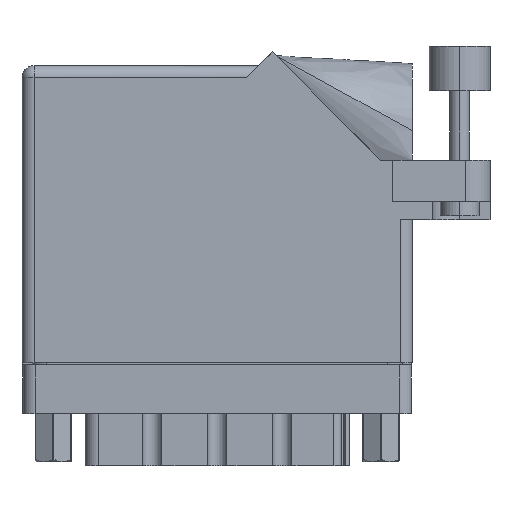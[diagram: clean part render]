
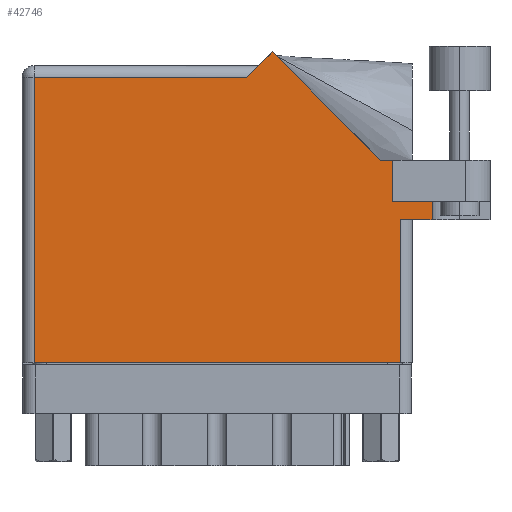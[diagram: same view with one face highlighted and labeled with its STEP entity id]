
A CAD part, front view. The second image highlights one B-rep face of the part: STEP entity #42746.
In plain terms, the highlighted face is planar.
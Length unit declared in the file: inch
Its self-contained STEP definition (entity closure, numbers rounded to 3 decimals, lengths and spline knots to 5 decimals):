
#1535 = CARTESIAN_POINT ( 'NONE',  ( 1.155, 1.468, 0. ) ) ;
#1618 = VECTOR ( 'NONE', #23216, 39.37008 ) ;
#1733 = PLANE ( 'NONE',  #25027 ) ;
#2465 = CARTESIAN_POINT ( 'NONE',  ( 1.217, 1.53, 0. ) ) ;
#3577 = VECTOR ( 'NONE', #14190, 39.37008 ) ;
#3691 = CARTESIAN_POINT ( 'NONE',  ( 1.84442, 1.044, 0. ) ) ;
#4006 = LINE ( 'NONE', #43678, #33752 ) ;
#4543 = VERTEX_POINT ( 'NONE', #36850 ) ;
#5243 = DIRECTION ( 'NONE',  ( -1., 0., 0. ) ) ;
#6204 = EDGE_CURVE ( 'NONE', #18071, #45854, #47728, .T. ) ;
#6948 = EDGE_CURVE ( 'NONE', #42936, #18071, #4006, .T. ) ;
#7545 = ORIENTED_EDGE ( 'NONE', *, *, #11452, .T. ) ;
#8191 = ORIENTED_EDGE ( 'NONE', *, *, #13982, .T. ) ;
#8495 = VECTOR ( 'NONE', #10688, 39.37008 ) ;
#9324 = ORIENTED_EDGE ( 'NONE', *, *, #23340, .F. ) ;
#9663 = LINE ( 'NONE', #29232, #18688 ) ;
#10382 = CARTESIAN_POINT ( 'NONE',  ( 2.1115, 1.16177, 0. ) ) ;
#10423 = VECTOR ( 'NONE', #29510, 39.37008 ) ;
#10688 = DIRECTION ( 'NONE',  ( 0., -1., 0. ) ) ;
#10839 = CARTESIAN_POINT ( 'NONE',  ( 0., 0., 0. ) ) ;
#11452 = EDGE_CURVE ( 'NONE', #45854, #25135, #19325, .T. ) ;
#12275 = EDGE_CURVE ( 'NONE', #35426, #27880, #9663, .T. ) ;
#13713 = DIRECTION ( 'NONE',  ( -1., 0., 0. ) ) ;
#13982 = EDGE_CURVE ( 'NONE', #35426, #42936, #41427, .T. ) ;
#14123 = DIRECTION ( 'NONE',  ( 0., 0., -1. ) ) ;
#14190 = DIRECTION ( 'NONE',  ( -0.707, -0.707, 0. ) ) ;
#15626 = CARTESIAN_POINT ( 'NONE',  ( 2.1115, 0.737, 0. ) ) ;
#17473 = VECTOR ( 'NONE', #19824, 39.37008 ) ;
#17929 = VECTOR ( 'NONE', #42366, 39.37008 ) ;
#17987 = DIRECTION ( 'NONE',  ( -1., 0., 0. ) ) ;
#18071 = VERTEX_POINT ( 'NONE', #38357 ) ;
#18688 = VECTOR ( 'NONE', #44945, 39.37008 ) ;
#19325 = LINE ( 'NONE', #2465, #3577 ) ;
#19680 = ORIENTED_EDGE ( 'NONE', *, *, #31225, .T. ) ;
#19824 = DIRECTION ( 'NONE',  ( 0., 1., 0. ) ) ;
#19980 = CARTESIAN_POINT ( 'NONE',  ( 1.91, 0.831, 0. ) ) ;
#21024 = EDGE_CURVE ( 'NONE', #4543, #29159, #24658, .T. ) ;
#22204 = ORIENTED_EDGE ( 'NONE', *, *, #6204, .T. ) ;
#23216 = DIRECTION ( 'NONE',  ( -0.707, 0.707, 0. ) ) ;
#23340 = EDGE_CURVE ( 'NONE', #27880, #29159, #29975, .T. ) ;
#24658 = LINE ( 'NONE', #46274, #17929 ) ;
#24709 = FACE_OUTER_BOUND ( 'NONE', #35248, .T. ) ;
#25027 = AXIS2_PLACEMENT_3D ( 'NONE', #32777, #14123, #17987 ) ;
#25135 = VERTEX_POINT ( 'NONE', #1535 ) ;
#25225 = EDGE_CURVE ( 'NONE', #42464, #33213, #40710, .T. ) ;
#26280 = CARTESIAN_POINT ( 'NONE',  ( 0., 1.468, 0. ) ) ;
#27232 = LINE ( 'NONE', #26280, #27827 ) ;
#27825 = CARTESIAN_POINT ( 'NONE',  ( 0.062, 0., 0. ) ) ;
#27827 = VECTOR ( 'NONE', #13713, 39.37008 ) ;
#27880 = VERTEX_POINT ( 'NONE', #39480 ) ;
#27953 = CARTESIAN_POINT ( 'NONE',  ( 0.062, 0., 0. ) ) ;
#28013 = CARTESIAN_POINT ( 'NONE',  ( 1.91, 0.831, 0. ) ) ;
#29159 = VERTEX_POINT ( 'NONE', #15626 ) ;
#29232 = CARTESIAN_POINT ( 'NONE',  ( 1.91, 0.831, 0. ) ) ;
#29402 = ORIENTED_EDGE ( 'NONE', *, *, #41650, .T. ) ;
#29510 = DIRECTION ( 'NONE',  ( 1., 0., 0. ) ) ;
#29975 = LINE ( 'NONE', #10382, #40800 ) ;
#30080 = CARTESIAN_POINT ( 'NONE',  ( 1.91, 1.044, 0. ) ) ;
#30337 = ORIENTED_EDGE ( 'NONE', *, *, #21024, .T. ) ;
#30879 = CARTESIAN_POINT ( 'NONE',  ( 1.28771, 1.60071, 0. ) ) ;
#31225 = EDGE_CURVE ( 'NONE', #38385, #42464, #44227, .T. ) ;
#31890 = ORIENTED_EDGE ( 'NONE', *, *, #25225, .T. ) ;
#32777 = CARTESIAN_POINT ( 'NONE',  ( 0., 1.53, 0. ) ) ;
#33213 = VERTEX_POINT ( 'NONE', #44200 ) ;
#33576 = DIRECTION ( 'NONE',  ( 0., -1., 0. ) ) ;
#33752 = VECTOR ( 'NONE', #5243, 39.37008 ) ;
#34679 = CARTESIAN_POINT ( 'NONE',  ( 0.062, 1.468, 0. ) ) ;
#35248 = EDGE_LOOP ( 'NONE', ( #31890, #38006, #30337, #9324, #44285, #8191, #39611, #22204, #7545, #29402, #19680 ) ) ;
#35426 = VERTEX_POINT ( 'NONE', #19980 ) ;
#35747 = CARTESIAN_POINT ( 'NONE',  ( 1.948, 0.737, 0. ) ) ;
#36850 = CARTESIAN_POINT ( 'NONE',  ( 1.948, 0.737, 0. ) ) ;
#37785 = VECTOR ( 'NONE', #47267, 39.37008 ) ;
#38006 = ORIENTED_EDGE ( 'NONE', *, *, #41460, .T. ) ;
#38357 = CARTESIAN_POINT ( 'NONE',  ( 1.84442, 1.044, 0. ) ) ;
#38385 = VERTEX_POINT ( 'NONE', #34679 ) ;
#39480 = CARTESIAN_POINT ( 'NONE',  ( 2.1115, 0.831, 0. ) ) ;
#39611 = ORIENTED_EDGE ( 'NONE', *, *, #6948, .T. ) ;
#40710 = LINE ( 'NONE', #10839, #10423 ) ;
#40800 = VECTOR ( 'NONE', #33576, 39.37008 ) ;
#41427 = LINE ( 'NONE', #28013, #37785 ) ;
#41460 = EDGE_CURVE ( 'NONE', #33213, #4543, #41774, .T. ) ;
#41650 = EDGE_CURVE ( 'NONE', #25135, #38385, #27232, .T. ) ;
#41774 = LINE ( 'NONE', #35747, #17473 ) ;
#42366 = DIRECTION ( 'NONE',  ( 1., 0., 0. ) ) ;
#42464 = VERTEX_POINT ( 'NONE', #27953 ) ;
#42746 = ADVANCED_FACE ( 'NONE', ( #24709 ), #1733, .F. ) ;
#42936 = VERTEX_POINT ( 'NONE', #30080 ) ;
#43678 = CARTESIAN_POINT ( 'NONE',  ( 2.41, 1.044, 0. ) ) ;
#44200 = CARTESIAN_POINT ( 'NONE',  ( 1.948, 0., 0. ) ) ;
#44227 = LINE ( 'NONE', #27825, #8495 ) ;
#44285 = ORIENTED_EDGE ( 'NONE', *, *, #12275, .F. ) ;
#44945 = DIRECTION ( 'NONE',  ( 1., 0., 0. ) ) ;
#45854 = VERTEX_POINT ( 'NONE', #30879 ) ;
#46274 = CARTESIAN_POINT ( 'NONE',  ( 2.01, 0.737, 0. ) ) ;
#47267 = DIRECTION ( 'NONE',  ( 0., 1., 0. ) ) ;
#47728 = LINE ( 'NONE', #3691, #1618 ) ;
